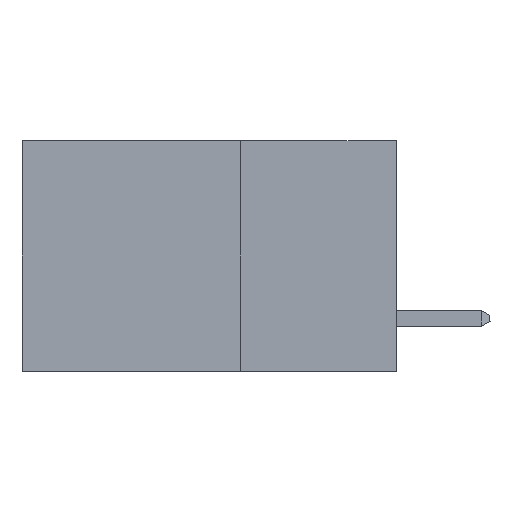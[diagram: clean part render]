
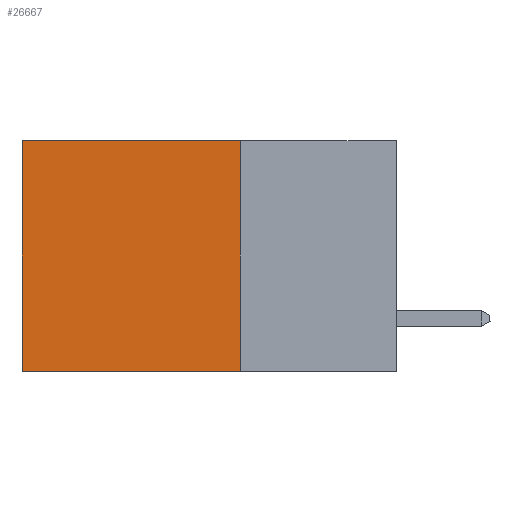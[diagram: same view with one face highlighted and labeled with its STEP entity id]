
A CAD part, left-side view. The second image highlights one B-rep face of the part: STEP entity #26667.
In plain terms, the highlighted planar face has unit normal (-1, 0, 0).
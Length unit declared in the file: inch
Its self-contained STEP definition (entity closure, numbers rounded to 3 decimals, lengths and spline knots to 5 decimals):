
#20 = LINE ( 'NONE', #29849, #12480 ) ;
#1125 = ORIENTED_EDGE ( 'NONE', *, *, #18605, .F. ) ;
#1198 = CARTESIAN_POINT ( 'NONE',  ( 0.298, 0.25, 0. ) ) ;
#1598 = DIRECTION ( 'NONE',  ( 0., 1., 0. ) ) ;
#1686 = LINE ( 'NONE', #25821, #14931 ) ;
#1904 = VERTEX_POINT ( 'NONE', #13196 ) ;
#2169 = AXIS2_PLACEMENT_3D ( 'NONE', #1198, #3713, #21064 ) ;
#2181 = VERTEX_POINT ( 'NONE', #3247 ) ;
#3247 = CARTESIAN_POINT ( 'NONE',  ( 0.298, 0.25, -0.37 ) ) ;
#3713 = DIRECTION ( 'NONE',  ( 1., 0., 0. ) ) ;
#3941 = EDGE_CURVE ( 'NONE', #1904, #6971, #20, .T. ) ;
#5133 = ORIENTED_EDGE ( 'NONE', *, *, #11795, .T. ) ;
#6971 = VERTEX_POINT ( 'NONE', #13545 ) ;
#9821 = VECTOR ( 'NONE', #1598, 39.37008 ) ;
#10604 = LINE ( 'NONE', #16390, #9821 ) ;
#11062 = DIRECTION ( 'NONE',  ( 0., 0., -1. ) ) ;
#11243 = VECTOR ( 'NONE', #25014, 39.37008 ) ;
#11795 = EDGE_CURVE ( 'NONE', #6971, #24672, #12009, .T. ) ;
#12009 = LINE ( 'NONE', #29783, #11243 ) ;
#12480 = VECTOR ( 'NONE', #27282, 39.37008 ) ;
#12926 = FACE_OUTER_BOUND ( 'NONE', #20019, .T. ) ;
#13196 = CARTESIAN_POINT ( 'NONE',  ( 0.298, 0.25, 0. ) ) ;
#13545 = CARTESIAN_POINT ( 'NONE',  ( 0.298, 0.6, 0. ) ) ;
#13764 = ORIENTED_EDGE ( 'NONE', *, *, #3941, .T. ) ;
#14931 = VECTOR ( 'NONE', #11062, 39.37008 ) ;
#16390 = CARTESIAN_POINT ( 'NONE',  ( 0.298, 0.25, -0.37 ) ) ;
#18498 = EDGE_CURVE ( 'NONE', #1904, #2181, #1686, .T. ) ;
#18605 = EDGE_CURVE ( 'NONE', #2181, #24672, #10604, .T. ) ;
#18624 = PLANE ( 'NONE',  #2169 ) ;
#20019 = EDGE_LOOP ( 'NONE', ( #5133, #1125, #26600, #13764 ) ) ;
#21064 = DIRECTION ( 'NONE',  ( 0., 0., -1. ) ) ;
#22545 = CARTESIAN_POINT ( 'NONE',  ( 0.298, 0.6, -0.37 ) ) ;
#24672 = VERTEX_POINT ( 'NONE', #22545 ) ;
#25014 = DIRECTION ( 'NONE',  ( 0., 0., -1. ) ) ;
#25821 = CARTESIAN_POINT ( 'NONE',  ( 0.298, 0.25, 0. ) ) ;
#26600 = ORIENTED_EDGE ( 'NONE', *, *, #18498, .F. ) ;
#26667 = ADVANCED_FACE ( 'NONE', ( #12926 ), #18624, .F. ) ;
#27282 = DIRECTION ( 'NONE',  ( 0., 1., 0. ) ) ;
#29783 = CARTESIAN_POINT ( 'NONE',  ( 0.298, 0.6, 0. ) ) ;
#29849 = CARTESIAN_POINT ( 'NONE',  ( 0.298, 0.25, 0. ) ) ;
